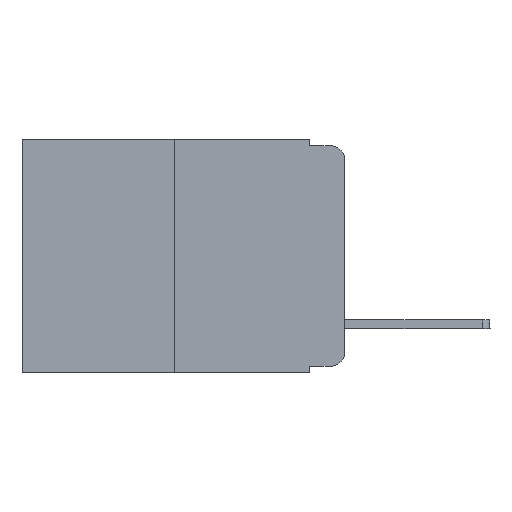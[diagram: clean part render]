
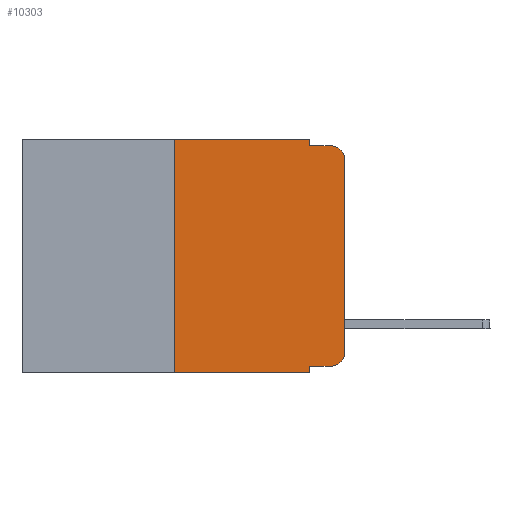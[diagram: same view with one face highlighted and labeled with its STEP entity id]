
A CAD part, left-side view. The second image highlights one B-rep face of the part: STEP entity #10303.
In plain terms, the highlighted planar face has unit normal (-1, 0, 0).
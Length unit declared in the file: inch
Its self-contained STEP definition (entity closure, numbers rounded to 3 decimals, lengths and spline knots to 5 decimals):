
#250 = CIRCLE ( 'NONE', #6936, 0.02 ) ;
#506 = PLANE ( 'NONE',  #22496 ) ;
#612 = CARTESIAN_POINT ( 'NONE',  ( 0., 0.051, -0.343 ) ) ;
#806 = EDGE_CURVE ( 'NONE', #15651, #23412, #16597, .T. ) ;
#946 = VERTEX_POINT ( 'NONE', #612 ) ;
#1268 = CARTESIAN_POINT ( 'NONE',  ( 0., 0.051, -0.333 ) ) ;
#1350 = DIRECTION ( 'NONE',  ( 0., -1., 0. ) ) ;
#1423 = CARTESIAN_POINT ( 'NONE',  ( 0., 0., -0.313 ) ) ;
#1607 = EDGE_CURVE ( 'NONE', #5848, #10500, #3102, .T. ) ;
#1626 = VECTOR ( 'NONE', #15567, 39.37008 ) ;
#1923 = LINE ( 'NONE', #22725, #15125 ) ;
#1995 = CARTESIAN_POINT ( 'NONE',  ( 0., 0.25, 0. ) ) ;
#2438 = LINE ( 'NONE', #22699, #1626 ) ;
#3102 = LINE ( 'NONE', #1268, #11107 ) ;
#3510 = ORIENTED_EDGE ( 'NONE', *, *, #18338, .T. ) ;
#3770 = ORIENTED_EDGE ( 'NONE', *, *, #23188, .T. ) ;
#4353 = CARTESIAN_POINT ( 'NONE',  ( 0., 0.25, -0.343 ) ) ;
#4741 = EDGE_CURVE ( 'NONE', #10500, #7238, #250, .T. ) ;
#5443 = CARTESIAN_POINT ( 'NONE',  ( 0., 0., 0. ) ) ;
#5848 = VERTEX_POINT ( 'NONE', #8304 ) ;
#5901 = DIRECTION ( 'NONE',  ( 0., -1., 0. ) ) ;
#6167 = CIRCLE ( 'NONE', #12947, 0.02 ) ;
#6568 = CARTESIAN_POINT ( 'NONE',  ( 0., 0.473, -0.343 ) ) ;
#6869 = DIRECTION ( 'NONE',  ( 0., 0., -1. ) ) ;
#6936 = AXIS2_PLACEMENT_3D ( 'NONE', #15897, #17928, #6869 ) ;
#7201 = ORIENTED_EDGE ( 'NONE', *, *, #1607, .T. ) ;
#7238 = VERTEX_POINT ( 'NONE', #1423 ) ;
#7519 = LINE ( 'NONE', #12521, #23716 ) ;
#7699 = EDGE_CURVE ( 'NONE', #16241, #15651, #2438, .T. ) ;
#8039 = ORIENTED_EDGE ( 'NONE', *, *, #4741, .T. ) ;
#8178 = CARTESIAN_POINT ( 'NONE',  ( 0., 0.02, -0.333 ) ) ;
#8203 = CARTESIAN_POINT ( 'NONE',  ( 0., 0.051, 0. ) ) ;
#8252 = CARTESIAN_POINT ( 'NONE',  ( 0., 0.02, -0.03 ) ) ;
#8304 = CARTESIAN_POINT ( 'NONE',  ( 0., 0.051, -0.333 ) ) ;
#8486 = VECTOR ( 'NONE', #18037, 39.37008 ) ;
#9294 = EDGE_CURVE ( 'NONE', #5848, #946, #7519, .T. ) ;
#9453 = DIRECTION ( 'NONE',  ( 0., 0., -1. ) ) ;
#9819 = EDGE_CURVE ( 'NONE', #16241, #946, #15877, .T. ) ;
#9866 = CARTESIAN_POINT ( 'NONE',  ( 0., 0.473, 0. ) ) ;
#10303 = ADVANCED_FACE ( 'NONE', ( #16708 ), #506, .F. ) ;
#10500 = VERTEX_POINT ( 'NONE', #8178 ) ;
#10716 = ORIENTED_EDGE ( 'NONE', *, *, #9819, .T. ) ;
#10964 = VECTOR ( 'NONE', #5901, 39.37008 ) ;
#11107 = VECTOR ( 'NONE', #1350, 39.37008 ) ;
#11413 = DIRECTION ( 'NONE',  ( 1., 0., 0. ) ) ;
#12521 = CARTESIAN_POINT ( 'NONE',  ( 0., 0.051, 0. ) ) ;
#12943 = VERTEX_POINT ( 'NONE', #15239 ) ;
#12947 = AXIS2_PLACEMENT_3D ( 'NONE', #8252, #13760, #19259 ) ;
#13192 = VECTOR ( 'NONE', #15364, 39.37008 ) ;
#13625 = ORIENTED_EDGE ( 'NONE', *, *, #14773, .F. ) ;
#13760 = DIRECTION ( 'NONE',  ( -1., 0., 0. ) ) ;
#14379 = DIRECTION ( 'NONE',  ( 0., 0., -1. ) ) ;
#14773 = EDGE_CURVE ( 'NONE', #23412, #20477, #1923, .T. ) ;
#15125 = VECTOR ( 'NONE', #9453, 39.37008 ) ;
#15177 = LINE ( 'NONE', #5443, #15438 ) ;
#15239 = CARTESIAN_POINT ( 'NONE',  ( 0., 0.02, -0.01 ) ) ;
#15261 = CARTESIAN_POINT ( 'NONE',  ( 0., 0., -0.03 ) ) ;
#15364 = DIRECTION ( 'NONE',  ( 0., -1., 0. ) ) ;
#15438 = VECTOR ( 'NONE', #22289, 39.37008 ) ;
#15567 = DIRECTION ( 'NONE',  ( 0., 0., 1. ) ) ;
#15651 = VERTEX_POINT ( 'NONE', #1995 ) ;
#15877 = LINE ( 'NONE', #6568, #10964 ) ;
#15897 = CARTESIAN_POINT ( 'NONE',  ( 0., 0.02, -0.313 ) ) ;
#16241 = VERTEX_POINT ( 'NONE', #4353 ) ;
#16404 = CARTESIAN_POINT ( 'NONE',  ( 0., 0.473, 0. ) ) ;
#16597 = LINE ( 'NONE', #16404, #8486 ) ;
#16620 = VERTEX_POINT ( 'NONE', #15261 ) ;
#16708 = FACE_OUTER_BOUND ( 'NONE', #21027, .T. ) ;
#16911 = DIRECTION ( 'NONE',  ( 0., 0., -1. ) ) ;
#17928 = DIRECTION ( 'NONE',  ( -1., 0., 0. ) ) ;
#18037 = DIRECTION ( 'NONE',  ( 0., -1., 0. ) ) ;
#18338 = EDGE_CURVE ( 'NONE', #16620, #12943, #6167, .T. ) ;
#18929 = ORIENTED_EDGE ( 'NONE', *, *, #7699, .F. ) ;
#19259 = DIRECTION ( 'NONE',  ( 0., 0., -1. ) ) ;
#20477 = VERTEX_POINT ( 'NONE', #23486 ) ;
#20916 = ORIENTED_EDGE ( 'NONE', *, *, #21974, .F. ) ;
#21027 = EDGE_LOOP ( 'NONE', ( #3770, #3510, #20916, #13625, #22164, #18929, #10716, #23316, #7201, #8039 ) ) ;
#21134 = CARTESIAN_POINT ( 'NONE',  ( 0., 0.051, -0.01 ) ) ;
#21974 = EDGE_CURVE ( 'NONE', #20477, #12943, #22442, .T. ) ;
#22164 = ORIENTED_EDGE ( 'NONE', *, *, #806, .F. ) ;
#22289 = DIRECTION ( 'NONE',  ( 0., 0., 1. ) ) ;
#22442 = LINE ( 'NONE', #21134, #13192 ) ;
#22496 = AXIS2_PLACEMENT_3D ( 'NONE', #9866, #11413, #16911 ) ;
#22699 = CARTESIAN_POINT ( 'NONE',  ( 0., 0.25, 0. ) ) ;
#22725 = CARTESIAN_POINT ( 'NONE',  ( 0., 0.051, 0. ) ) ;
#23188 = EDGE_CURVE ( 'NONE', #7238, #16620, #15177, .T. ) ;
#23316 = ORIENTED_EDGE ( 'NONE', *, *, #9294, .F. ) ;
#23412 = VERTEX_POINT ( 'NONE', #8203 ) ;
#23486 = CARTESIAN_POINT ( 'NONE',  ( 0., 0.051, -0.01 ) ) ;
#23716 = VECTOR ( 'NONE', #14379, 39.37008 ) ;
